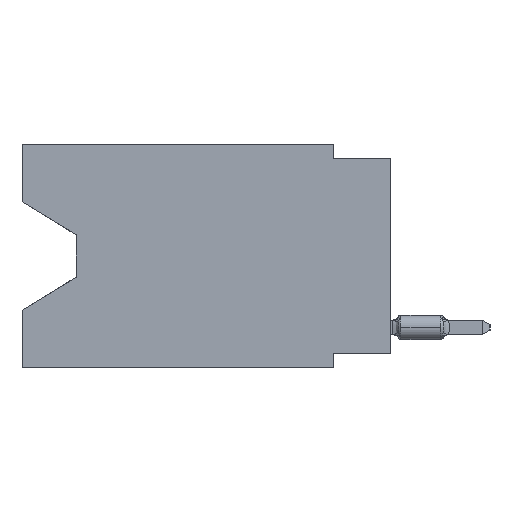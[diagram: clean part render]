
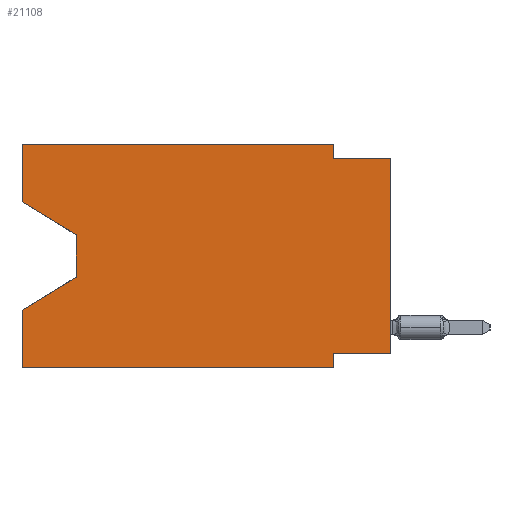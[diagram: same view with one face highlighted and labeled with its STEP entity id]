
A CAD part, left-side view. The second image highlights one B-rep face of the part: STEP entity #21108.
In plain terms, the highlighted planar face has unit normal (-1, 0, 0).
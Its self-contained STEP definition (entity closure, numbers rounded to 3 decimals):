
#371 = CARTESIAN_POINT ( 'NONE',  ( 0., 16.383, 0. ) ) ;
#682 = VECTOR ( 'NONE', #48434, 1000. ) ;
#1182 = VERTEX_POINT ( 'NONE', #40967 ) ;
#1922 = ORIENTED_EDGE ( 'NONE', *, *, #44700, .T. ) ;
#3744 = CARTESIAN_POINT ( 'NONE',  ( 0., 16.383, -9.906 ) ) ;
#3789 = DIRECTION ( 'NONE',  ( 0., 0.855, -0.519 ) ) ;
#3916 = ORIENTED_EDGE ( 'NONE', *, *, #39114, .F. ) ;
#5271 = LINE ( 'NONE', #67337, #36560 ) ;
#5630 = DIRECTION ( 'NONE',  ( 0., 0., 1. ) ) ;
#5922 = CARTESIAN_POINT ( 'NONE',  ( 0., 16.383, 0. ) ) ;
#5934 = DIRECTION ( 'NONE',  ( 0., -1., 0. ) ) ;
#6802 = VECTOR ( 'NONE', #46865, 1000. ) ;
#7496 = EDGE_CURVE ( 'NONE', #48129, #1182, #9243, .T. ) ;
#8047 = CARTESIAN_POINT ( 'NONE',  ( 0., 16.383, -2.546 ) ) ;
#8135 = LINE ( 'NONE', #25471, #34570 ) ;
#9243 = LINE ( 'NONE', #48023, #46861 ) ;
#10074 = EDGE_CURVE ( 'NONE', #14629, #36089, #37792, .T. ) ;
#10555 = LINE ( 'NONE', #43436, #43636 ) ;
#11313 = EDGE_CURVE ( 'NONE', #42420, #55310, #5271, .T. ) ;
#12753 = DIRECTION ( 'NONE',  ( 0., 0., -1. ) ) ;
#13003 = VERTEX_POINT ( 'NONE', #5922 ) ;
#13945 = EDGE_CURVE ( 'NONE', #42420, #17223, #54363, .T. ) ;
#14629 = VERTEX_POINT ( 'NONE', #59321 ) ;
#15177 = VECTOR ( 'NONE', #17487, 1000. ) ;
#15607 = DIRECTION ( 'NONE',  ( 0., 0., 1. ) ) ;
#16618 = DIRECTION ( 'NONE',  ( 0., -1., 0. ) ) ;
#17223 = VERTEX_POINT ( 'NONE', #52178 ) ;
#17487 = DIRECTION ( 'NONE',  ( 0., 0., -1. ) ) ;
#19501 = ORIENTED_EDGE ( 'NONE', *, *, #58451, .T. ) ;
#19583 = DIRECTION ( 'NONE',  ( 0., -0.855, -0.519 ) ) ;
#20289 = DIRECTION ( 'NONE',  ( 0., 0., 1. ) ) ;
#21108 = ADVANCED_FACE ( 'NONE', ( #25769 ), #32429, .F. ) ;
#21744 = CARTESIAN_POINT ( 'NONE',  ( 0., 2.54, -9.271 ) ) ;
#21946 = LINE ( 'NONE', #45574, #15177 ) ;
#22210 = EDGE_CURVE ( 'NONE', #48129, #13003, #8135, .T. ) ;
#23449 = CARTESIAN_POINT ( 'NONE',  ( 0., 13.97, -4.013 ) ) ;
#23817 = LINE ( 'NONE', #23449, #43150 ) ;
#24182 = VECTOR ( 'NONE', #5934, 1000. ) ;
#24335 = CARTESIAN_POINT ( 'NONE',  ( 0., 0., -9.271 ) ) ;
#24736 = VERTEX_POINT ( 'NONE', #36937 ) ;
#25471 = CARTESIAN_POINT ( 'NONE',  ( 0., 16.383, 0. ) ) ;
#25769 = FACE_OUTER_BOUND ( 'NONE', #60458, .T. ) ;
#25852 = VERTEX_POINT ( 'NONE', #35235 ) ;
#26319 = CARTESIAN_POINT ( 'NONE',  ( 0., 13.97, -5.893 ) ) ;
#30605 = VECTOR ( 'NONE', #16618, 1000. ) ;
#30953 = CARTESIAN_POINT ( 'NONE',  ( 0., 0., -0.635 ) ) ;
#31058 = ORIENTED_EDGE ( 'NONE', *, *, #22210, .F. ) ;
#31317 = DIRECTION ( 'NONE',  ( 0., 0., -1. ) ) ;
#32429 = PLANE ( 'NONE',  #52084 ) ;
#32898 = ORIENTED_EDGE ( 'NONE', *, *, #63834, .F. ) ;
#34570 = VECTOR ( 'NONE', #20289, 1000. ) ;
#35235 = CARTESIAN_POINT ( 'NONE',  ( 0., 0., -9.271 ) ) ;
#35839 = EDGE_CURVE ( 'NONE', #25852, #36089, #48474, .T. ) ;
#36036 = EDGE_CURVE ( 'NONE', #25852, #47895, #57977, .T. ) ;
#36089 = VERTEX_POINT ( 'NONE', #30953 ) ;
#36499 = DIRECTION ( 'NONE',  ( 1., 0., 0. ) ) ;
#36560 = VECTOR ( 'NONE', #5630, 1000. ) ;
#36937 = CARTESIAN_POINT ( 'NONE',  ( 0., 2.54, 0. ) ) ;
#37792 = LINE ( 'NONE', #60342, #30605 ) ;
#38633 = VECTOR ( 'NONE', #15607, 1000. ) ;
#38805 = LINE ( 'NONE', #371, #24182 ) ;
#39114 = EDGE_CURVE ( 'NONE', #24736, #14629, #10555, .T. ) ;
#39659 = CARTESIAN_POINT ( 'NONE',  ( 0., 13.97, -5.893 ) ) ;
#40967 = CARTESIAN_POINT ( 'NONE',  ( 0., 13.97, -4.013 ) ) ;
#41001 = ORIENTED_EDGE ( 'NONE', *, *, #11313, .F. ) ;
#42420 = VERTEX_POINT ( 'NONE', #66115 ) ;
#43150 = VECTOR ( 'NONE', #12753, 1000. ) ;
#43299 = CARTESIAN_POINT ( 'NONE',  ( 0., 0., 0. ) ) ;
#43436 = CARTESIAN_POINT ( 'NONE',  ( 0., 2.54, 0. ) ) ;
#43636 = VECTOR ( 'NONE', #56371, 1000. ) ;
#44700 = EDGE_CURVE ( 'NONE', #62593, #55310, #60316, .T. ) ;
#45574 = CARTESIAN_POINT ( 'NONE',  ( 0., 2.54, -9.906 ) ) ;
#45780 = ORIENTED_EDGE ( 'NONE', *, *, #35839, .T. ) ;
#46358 = EDGE_CURVE ( 'NONE', #13003, #24736, #38805, .T. ) ;
#46861 = VECTOR ( 'NONE', #19583, 1000. ) ;
#46865 = DIRECTION ( 'NONE',  ( 0., 1., 0. ) ) ;
#47895 = VERTEX_POINT ( 'NONE', #21744 ) ;
#47943 = ORIENTED_EDGE ( 'NONE', *, *, #10074, .F. ) ;
#48023 = CARTESIAN_POINT ( 'NONE',  ( 0., 16.383, -2.546 ) ) ;
#48129 = VERTEX_POINT ( 'NONE', #8047 ) ;
#48434 = DIRECTION ( 'NONE',  ( 0., -1., 0. ) ) ;
#48474 = LINE ( 'NONE', #43299, #38633 ) ;
#48865 = CARTESIAN_POINT ( 'NONE',  ( 0., 16.383, -7.36 ) ) ;
#49911 = VECTOR ( 'NONE', #3789, 1000. ) ;
#52084 = AXIS2_PLACEMENT_3D ( 'NONE', #65679, #36499, #31317 ) ;
#52178 = CARTESIAN_POINT ( 'NONE',  ( 0., 2.54, -9.906 ) ) ;
#53803 = ORIENTED_EDGE ( 'NONE', *, *, #7496, .T. ) ;
#54363 = LINE ( 'NONE', #3744, #682 ) ;
#55310 = VERTEX_POINT ( 'NONE', #48865 ) ;
#55497 = ORIENTED_EDGE ( 'NONE', *, *, #46358, .F. ) ;
#56371 = DIRECTION ( 'NONE',  ( 0., 0., -1. ) ) ;
#57679 = ORIENTED_EDGE ( 'NONE', *, *, #13945, .T. ) ;
#57977 = LINE ( 'NONE', #24335, #6802 ) ;
#58451 = EDGE_CURVE ( 'NONE', #1182, #62593, #23817, .T. ) ;
#59321 = CARTESIAN_POINT ( 'NONE',  ( 0., 2.54, -0.635 ) ) ;
#60316 = LINE ( 'NONE', #26319, #49911 ) ;
#60342 = CARTESIAN_POINT ( 'NONE',  ( 0., 0., -0.635 ) ) ;
#60458 = EDGE_LOOP ( 'NONE', ( #53803, #19501, #1922, #41001, #57679, #32898, #64685, #45780, #47943, #3916, #55497, #31058 ) ) ;
#62593 = VERTEX_POINT ( 'NONE', #39659 ) ;
#63834 = EDGE_CURVE ( 'NONE', #47895, #17223, #21946, .T. ) ;
#64685 = ORIENTED_EDGE ( 'NONE', *, *, #36036, .F. ) ;
#65679 = CARTESIAN_POINT ( 'NONE',  ( 0., 16.383, 0. ) ) ;
#66115 = CARTESIAN_POINT ( 'NONE',  ( 0., 16.383, -9.906 ) ) ;
#67337 = CARTESIAN_POINT ( 'NONE',  ( 0., 16.383, 0. ) ) ;
